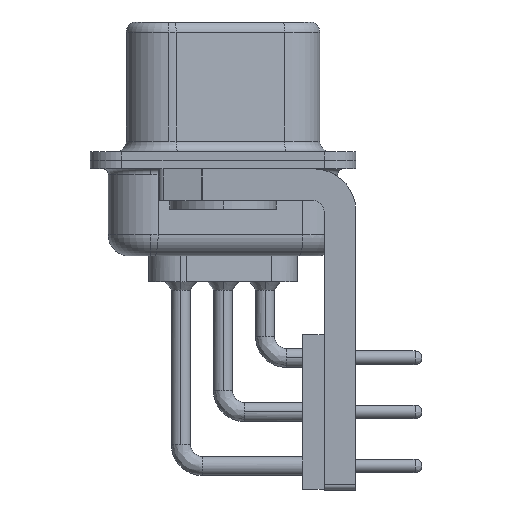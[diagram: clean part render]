
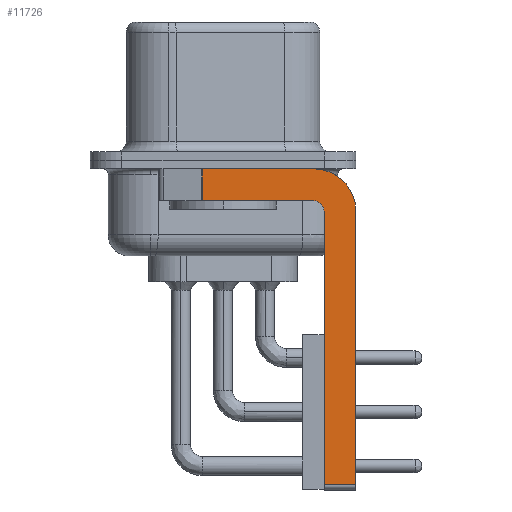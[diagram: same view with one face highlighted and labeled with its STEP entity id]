
A CAD part, left-side view. The second image highlights one B-rep face of the part: STEP entity #11726.
In plain terms, the highlighted planar face has unit normal (-1, 0, 0).
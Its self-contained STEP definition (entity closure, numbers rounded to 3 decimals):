
#666 = ORIENTED_EDGE ( 'NONE', *, *, #15021, .T. ) ;
#920 = CARTESIAN_POINT ( 'NONE',  ( -2.9, -6.25, -15.25 ) ) ;
#2244 = LINE ( 'NONE', #9446, #20054 ) ;
#2632 = DIRECTION ( 'NONE',  ( 0., 0., -1. ) ) ;
#4496 = VECTOR ( 'NONE', #27793, 1000. ) ;
#4502 = CARTESIAN_POINT ( 'NONE',  ( -2.9, -4.25, -2.4 ) ) ;
#4603 = CARTESIAN_POINT ( 'NONE',  ( -2.9, -4.25, -1.9 ) ) ;
#4733 = CARTESIAN_POINT ( 'NONE',  ( -2.9, -4.25, -1.9 ) ) ;
#4996 = VECTOR ( 'NONE', #18907, 1000. ) ;
#5103 = DIRECTION ( 'NONE',  ( -1., 0., 0. ) ) ;
#5841 = VECTOR ( 'NONE', #26492, 1000. ) ;
#6162 = AXIS2_PLACEMENT_3D ( 'NONE', #4502, #21368, #6951 ) ;
#6225 = ORIENTED_EDGE ( 'NONE', *, *, #16908, .F. ) ;
#6708 = VERTEX_POINT ( 'NONE', #6971 ) ;
#6951 = DIRECTION ( 'NONE',  ( 0., 0., -1. ) ) ;
#6971 = CARTESIAN_POINT ( 'NONE',  ( -2.9, -4.75, -15.25 ) ) ;
#7109 = CARTESIAN_POINT ( 'NONE',  ( -2.9, -4.25, -0.4 ) ) ;
#7391 = FACE_OUTER_BOUND ( 'NONE', #28750, .T. ) ;
#7529 = DIRECTION ( 'NONE',  ( 0., 0., -1. ) ) ;
#9446 = CARTESIAN_POINT ( 'NONE',  ( -2.9, 0.978, -1.9 ) ) ;
#10871 = CARTESIAN_POINT ( 'NONE',  ( -2.9, -4.75, -2.4 ) ) ;
#10896 = CARTESIAN_POINT ( 'NONE',  ( -2.9, -4.25, -15.25 ) ) ;
#10977 = VERTEX_POINT ( 'NONE', #10871 ) ;
#10997 = LINE ( 'NONE', #10896, #4496 ) ;
#11627 = CIRCLE ( 'NONE', #18625, 0.5 ) ;
#11698 = CARTESIAN_POINT ( 'NONE',  ( -2.9, 3., -0.4 ) ) ;
#11726 = ADVANCED_FACE ( 'NONE', ( #7391 ), #14787, .F. ) ;
#11814 = ORIENTED_EDGE ( 'NONE', *, *, #20771, .T. ) ;
#12662 = VECTOR ( 'NONE', #7529, 1000. ) ;
#13435 = LINE ( 'NONE', #17120, #12662 ) ;
#13843 = CIRCLE ( 'NONE', #6162, 2. ) ;
#14209 = DIRECTION ( 'NONE',  ( 0., 0., -1. ) ) ;
#14787 = PLANE ( 'NONE',  #20953 ) ;
#15021 = EDGE_CURVE ( 'NONE', #30908, #28337, #2244, .T. ) ;
#16814 = VERTEX_POINT ( 'NONE', #4733 ) ;
#16908 = EDGE_CURVE ( 'NONE', #19587, #27913, #13435, .T. ) ;
#17120 = CARTESIAN_POINT ( 'NONE',  ( -2.9, -6.25, -2.4 ) ) ;
#17176 = DIRECTION ( 'NONE',  ( 1., 0., 0. ) ) ;
#17301 = ORIENTED_EDGE ( 'NONE', *, *, #27746, .F. ) ;
#17410 = EDGE_CURVE ( 'NONE', #23354, #19587, #13843, .T. ) ;
#17475 = EDGE_CURVE ( 'NONE', #16814, #28337, #26641, .T. ) ;
#17859 = LINE ( 'NONE', #11698, #4996 ) ;
#18036 = VECTOR ( 'NONE', #21964, 1000. ) ;
#18107 = ORIENTED_EDGE ( 'NONE', *, *, #22777, .F. ) ;
#18625 = AXIS2_PLACEMENT_3D ( 'NONE', #19566, #5103, #21981 ) ;
#18907 = DIRECTION ( 'NONE',  ( 0., -1., 0. ) ) ;
#19539 = LINE ( 'NONE', #26967, #18036 ) ;
#19566 = CARTESIAN_POINT ( 'NONE',  ( -2.9, -4.25, -2.4 ) ) ;
#19587 = VERTEX_POINT ( 'NONE', #24080 ) ;
#20035 = CARTESIAN_POINT ( 'NONE',  ( -2.9, 0.978, -1.9 ) ) ;
#20054 = VECTOR ( 'NONE', #14209, 1000. ) ;
#20771 = EDGE_CURVE ( 'NONE', #6708, #27913, #10997, .T. ) ;
#20815 = ORIENTED_EDGE ( 'NONE', *, *, #17410, .F. ) ;
#20953 = AXIS2_PLACEMENT_3D ( 'NONE', #31599, #17176, #2632 ) ;
#21368 = DIRECTION ( 'NONE',  ( 1., 0., 0. ) ) ;
#21964 = DIRECTION ( 'NONE',  ( 0., 0., 1. ) ) ;
#21981 = DIRECTION ( 'NONE',  ( 0., 0., 1. ) ) ;
#22118 = ORIENTED_EDGE ( 'NONE', *, *, #30801, .F. ) ;
#22777 = EDGE_CURVE ( 'NONE', #10977, #16814, #11627, .T. ) ;
#23354 = VERTEX_POINT ( 'NONE', #7109 ) ;
#24080 = CARTESIAN_POINT ( 'NONE',  ( -2.9, -6.25, -2.4 ) ) ;
#26492 = DIRECTION ( 'NONE',  ( 0., 1., 0. ) ) ;
#26641 = LINE ( 'NONE', #4603, #5841 ) ;
#26967 = CARTESIAN_POINT ( 'NONE',  ( -2.9, -4.75, -15.5 ) ) ;
#27746 = EDGE_CURVE ( 'NONE', #6708, #10977, #19539, .T. ) ;
#27793 = DIRECTION ( 'NONE',  ( 0., -1., 0. ) ) ;
#27913 = VERTEX_POINT ( 'NONE', #920 ) ;
#28337 = VERTEX_POINT ( 'NONE', #20035 ) ;
#28750 = EDGE_LOOP ( 'NONE', ( #22118, #666, #29928, #18107, #17301, #11814, #6225, #20815 ) ) ;
#29030 = CARTESIAN_POINT ( 'NONE',  ( -2.9, 0.978, -0.4 ) ) ;
#29928 = ORIENTED_EDGE ( 'NONE', *, *, #17475, .F. ) ;
#30801 = EDGE_CURVE ( 'NONE', #30908, #23354, #17859, .T. ) ;
#30908 = VERTEX_POINT ( 'NONE', #29030 ) ;
#31599 = CARTESIAN_POINT ( 'NONE',  ( -2.9, -4.25, -2.4 ) ) ;
